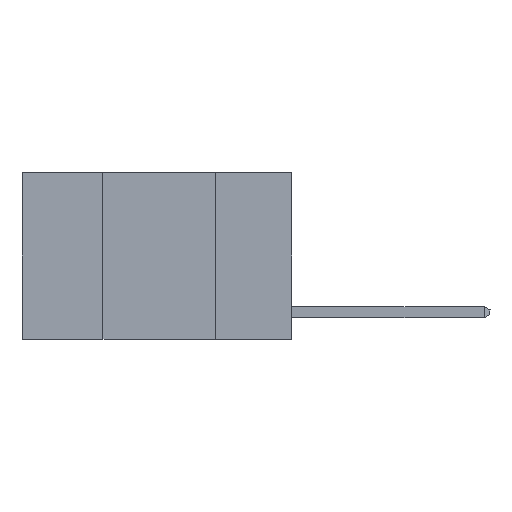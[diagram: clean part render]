
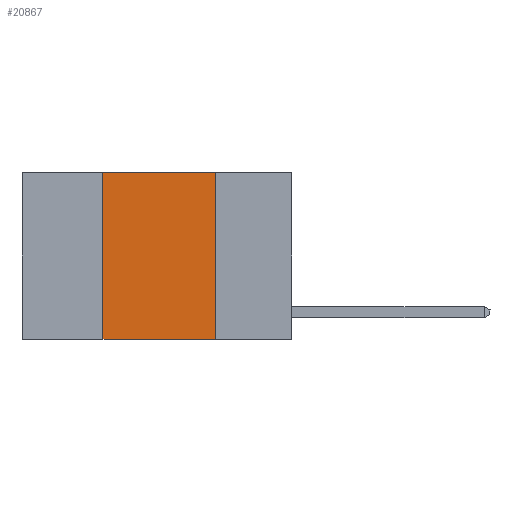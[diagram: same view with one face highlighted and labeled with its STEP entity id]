
A CAD part, left-side view. The second image highlights one B-rep face of the part: STEP entity #20867.
In plain terms, the highlighted planar face has unit normal (-1, 0, 0).
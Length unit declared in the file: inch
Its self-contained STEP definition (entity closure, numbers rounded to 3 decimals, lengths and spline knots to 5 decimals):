
#1177 = VECTOR ( 'NONE', #25378, 39.37008 ) ;
#1289 = CARTESIAN_POINT ( 'NONE',  ( 0., 0.6, 0. ) ) ;
#1899 = LINE ( 'NONE', #20986, #1177 ) ;
#2777 = CARTESIAN_POINT ( 'NONE',  ( 0., 0.17, 0. ) ) ;
#3353 = CARTESIAN_POINT ( 'NONE',  ( 0., 0.42, 0. ) ) ;
#4116 = CARTESIAN_POINT ( 'NONE',  ( 0., 0.42, -0.37 ) ) ;
#5158 = DIRECTION ( 'NONE',  ( 0., 0., -1. ) ) ;
#5994 = DIRECTION ( 'NONE',  ( 0., -1., 0. ) ) ;
#6606 = CARTESIAN_POINT ( 'NONE',  ( 0., 0.6, 0. ) ) ;
#7986 = CARTESIAN_POINT ( 'NONE',  ( 0., 0.17, -0.37 ) ) ;
#8426 = CARTESIAN_POINT ( 'NONE',  ( 0., 0.6, -0.37 ) ) ;
#8511 = VECTOR ( 'NONE', #5994, 39.37008 ) ;
#8967 = LINE ( 'NONE', #6606, #26019 ) ;
#9010 = FACE_OUTER_BOUND ( 'NONE', #17802, .T. ) ;
#10921 = PLANE ( 'NONE',  #19828 ) ;
#11392 = EDGE_CURVE ( 'NONE', #15845, #28619, #1899, .T. ) ;
#13051 = EDGE_CURVE ( 'NONE', #15845, #18124, #15693, .T. ) ;
#13377 = DIRECTION ( 'NONE',  ( 0., 0., -1. ) ) ;
#15693 = LINE ( 'NONE', #8426, #8511 ) ;
#15845 = VERTEX_POINT ( 'NONE', #4116 ) ;
#16621 = ORIENTED_EDGE ( 'NONE', *, *, #11392, .F. ) ;
#17802 = EDGE_LOOP ( 'NONE', ( #18119, #27611, #16621, #27094 ) ) ;
#17960 = LINE ( 'NONE', #2777, #29104 ) ;
#18119 = ORIENTED_EDGE ( 'NONE', *, *, #29786, .F. ) ;
#18124 = VERTEX_POINT ( 'NONE', #7986 ) ;
#18238 = VERTEX_POINT ( 'NONE', #24637 ) ;
#19828 = AXIS2_PLACEMENT_3D ( 'NONE', #1289, #27039, #13377 ) ;
#20867 = ADVANCED_FACE ( 'NONE', ( #9010 ), #10921, .F. ) ;
#20986 = CARTESIAN_POINT ( 'NONE',  ( 0., 0.42, 0. ) ) ;
#24637 = CARTESIAN_POINT ( 'NONE',  ( 0., 0.17, 0. ) ) ;
#25378 = DIRECTION ( 'NONE',  ( 0., 0., 1. ) ) ;
#26019 = VECTOR ( 'NONE', #29647, 39.37008 ) ;
#27039 = DIRECTION ( 'NONE',  ( 1., 0., 0. ) ) ;
#27094 = ORIENTED_EDGE ( 'NONE', *, *, #13051, .T. ) ;
#27611 = ORIENTED_EDGE ( 'NONE', *, *, #28914, .F. ) ;
#28619 = VERTEX_POINT ( 'NONE', #3353 ) ;
#28914 = EDGE_CURVE ( 'NONE', #28619, #18238, #8967, .T. ) ;
#29104 = VECTOR ( 'NONE', #5158, 39.37008 ) ;
#29647 = DIRECTION ( 'NONE',  ( 0., -1., 0. ) ) ;
#29786 = EDGE_CURVE ( 'NONE', #18238, #18124, #17960, .T. ) ;
